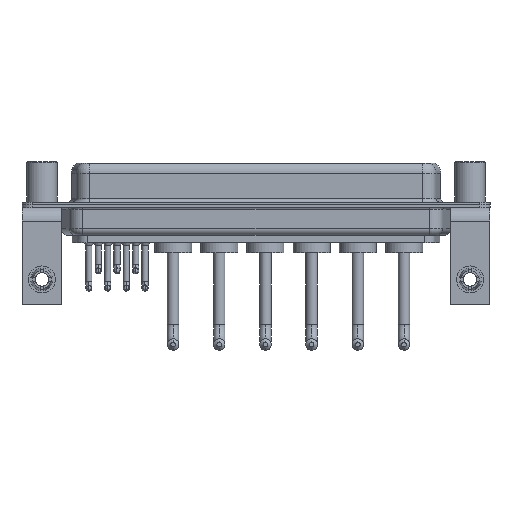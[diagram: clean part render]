
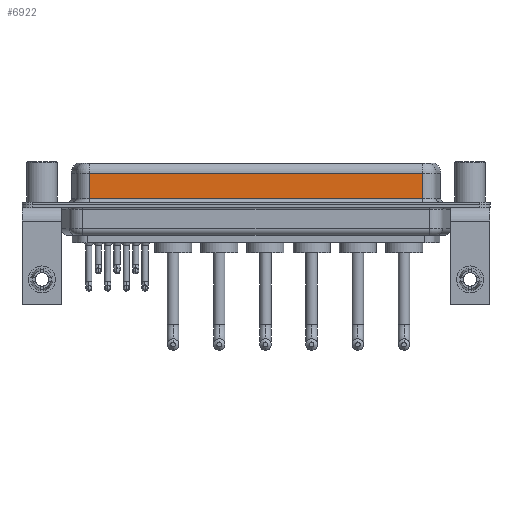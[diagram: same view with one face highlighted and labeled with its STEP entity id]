
A CAD part, front view. The second image highlights one B-rep face of the part: STEP entity #6922.
In plain terms, the highlighted planar face has unit normal (0, -1, 0).
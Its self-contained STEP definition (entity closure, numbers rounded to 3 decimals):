
#1100 = DIRECTION ( 'NONE',  ( 0., 0., 1. ) ) ;
#1183 = ORIENTED_EDGE ( 'NONE', *, *, #15719, .T. ) ;
#2718 = DIRECTION ( 'NONE',  ( 1., 0., 0. ) ) ;
#2818 = PLANE ( 'NONE',  #3780 ) ;
#3059 = EDGE_LOOP ( 'NONE', ( #13216, #1183, #7113, #3701 ) ) ;
#3601 = LINE ( 'NONE', #3943, #4553 ) ;
#3701 = ORIENTED_EDGE ( 'NONE', *, *, #18275, .T. ) ;
#3780 = AXIS2_PLACEMENT_3D ( 'NONE', #9758, #16738, #1100 ) ;
#3943 = CARTESIAN_POINT ( 'NONE',  ( 56.462, -3.95, 4.65 ) ) ;
#4553 = VECTOR ( 'NONE', #5523, 1000. ) ;
#4723 = DIRECTION ( 'NONE',  ( 0., 0., -1. ) ) ;
#5523 = DIRECTION ( 'NONE',  ( -1., 0., 0. ) ) ;
#6128 = CARTESIAN_POINT ( 'NONE',  ( 56.462, -3.95, 0.9 ) ) ;
#6650 = LINE ( 'NONE', #15342, #16996 ) ;
#6922 = ADVANCED_FACE ( 'NONE', ( #18442 ), #2818, .F. ) ;
#7113 = ORIENTED_EDGE ( 'NONE', *, *, #16940, .T. ) ;
#7330 = CARTESIAN_POINT ( 'NONE',  ( 56.462, -3.95, 4.65 ) ) ;
#9758 = CARTESIAN_POINT ( 'NONE',  ( 56.462, -3.95, 6.4 ) ) ;
#10026 = CARTESIAN_POINT ( 'NONE',  ( 7.038, -3.95, 4.65 ) ) ;
#10357 = VECTOR ( 'NONE', #18778, 1000. ) ;
#10450 = VECTOR ( 'NONE', #2718, 1000. ) ;
#12879 = CARTESIAN_POINT ( 'NONE',  ( 7.038, -3.95, 0.9 ) ) ;
#13216 = ORIENTED_EDGE ( 'NONE', *, *, #15571, .F. ) ;
#13510 = VERTEX_POINT ( 'NONE', #12879 ) ;
#14819 = LINE ( 'NONE', #6128, #10450 ) ;
#15342 = CARTESIAN_POINT ( 'NONE',  ( 7.038, -3.95, 6.4 ) ) ;
#15571 = EDGE_CURVE ( 'NONE', #17210, #20945, #18663, .T. ) ;
#15719 = EDGE_CURVE ( 'NONE', #17210, #16632, #3601, .T. ) ;
#16632 = VERTEX_POINT ( 'NONE', #10026 ) ;
#16738 = DIRECTION ( 'NONE',  ( 0., 1., 0. ) ) ;
#16940 = EDGE_CURVE ( 'NONE', #16632, #13510, #6650, .T. ) ;
#16996 = VECTOR ( 'NONE', #4723, 1000. ) ;
#17083 = CARTESIAN_POINT ( 'NONE',  ( 56.462, -3.95, 6.4 ) ) ;
#17210 = VERTEX_POINT ( 'NONE', #7330 ) ;
#17234 = CARTESIAN_POINT ( 'NONE',  ( 56.462, -3.95, 0.9 ) ) ;
#18275 = EDGE_CURVE ( 'NONE', #13510, #20945, #14819, .T. ) ;
#18442 = FACE_OUTER_BOUND ( 'NONE', #3059, .T. ) ;
#18663 = LINE ( 'NONE', #17083, #10357 ) ;
#18778 = DIRECTION ( 'NONE',  ( 0., 0., -1. ) ) ;
#20945 = VERTEX_POINT ( 'NONE', #17234 ) ;
